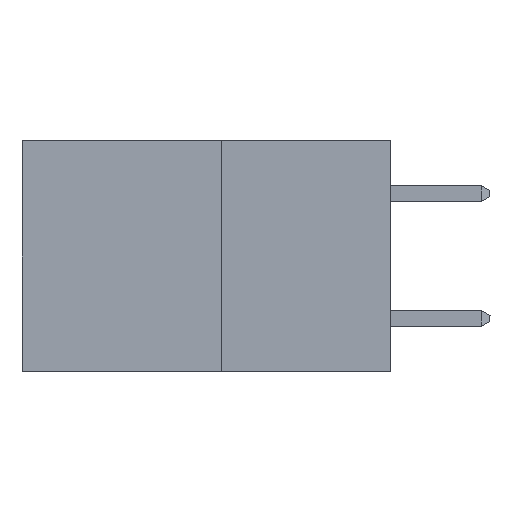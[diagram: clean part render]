
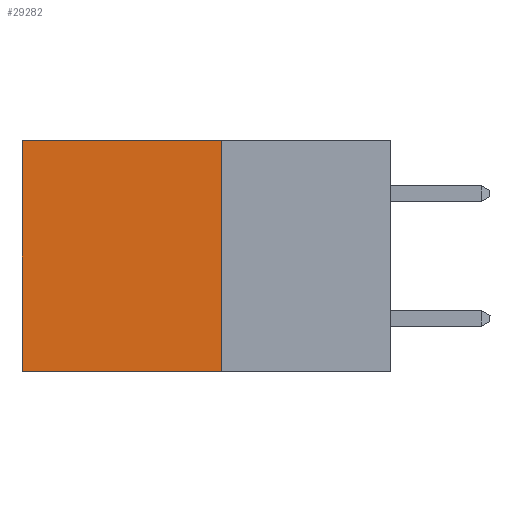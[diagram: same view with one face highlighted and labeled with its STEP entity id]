
A CAD part, left-side view. The second image highlights one B-rep face of the part: STEP entity #29282.
In plain terms, the highlighted planar face has unit normal (-1, 0, 0).
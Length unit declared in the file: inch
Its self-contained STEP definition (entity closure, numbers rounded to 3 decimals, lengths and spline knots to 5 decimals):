
#642 = CARTESIAN_POINT ( 'NONE',  ( 0.277, 0.59, -0.37 ) ) ;
#885 = CARTESIAN_POINT ( 'NONE',  ( 0.277, 0.27, -0.37 ) ) ;
#2436 = VERTEX_POINT ( 'NONE', #17858 ) ;
#3381 = DIRECTION ( 'NONE',  ( 0., 0., -1. ) ) ;
#3770 = AXIS2_PLACEMENT_3D ( 'NONE', #885, #18578, #3381 ) ;
#4627 = CARTESIAN_POINT ( 'NONE',  ( 0.277, 0.27, -0.37 ) ) ;
#4753 = CARTESIAN_POINT ( 'NONE',  ( 0.277, 0.27, 0. ) ) ;
#5964 = DIRECTION ( 'NONE',  ( 0., 0., -1. ) ) ;
#6075 = CARTESIAN_POINT ( 'NONE',  ( 0.277, 0.59, -0.37 ) ) ;
#6175 = VERTEX_POINT ( 'NONE', #27553 ) ;
#6670 = CARTESIAN_POINT ( 'NONE',  ( 0.277, 0.27, -0.37 ) ) ;
#7048 = LINE ( 'NONE', #6075, #19754 ) ;
#7184 = DIRECTION ( 'NONE',  ( 0., 0., -1. ) ) ;
#7358 = ORIENTED_EDGE ( 'NONE', *, *, #10114, .T. ) ;
#10114 = EDGE_CURVE ( 'NONE', #6175, #30348, #7048, .T. ) ;
#13541 = ORIENTED_EDGE ( 'NONE', *, *, #15179, .T. ) ;
#14337 = DIRECTION ( 'NONE',  ( 0., 1., 0. ) ) ;
#15179 = EDGE_CURVE ( 'NONE', #30487, #6175, #24378, .T. ) ;
#16260 = VECTOR ( 'NONE', #7184, 39.37008 ) ;
#17014 = ORIENTED_EDGE ( 'NONE', *, *, #24397, .F. ) ;
#17640 = VECTOR ( 'NONE', #27584, 39.37008 ) ;
#17770 = VECTOR ( 'NONE', #14337, 39.37008 ) ;
#17858 = CARTESIAN_POINT ( 'NONE',  ( 0.277, 0.27, -0.37 ) ) ;
#18578 = DIRECTION ( 'NONE',  ( 1., 0., 0. ) ) ;
#19754 = VECTOR ( 'NONE', #5964, 39.37008 ) ;
#20997 = PLANE ( 'NONE',  #3770 ) ;
#21864 = FACE_OUTER_BOUND ( 'NONE', #25273, .T. ) ;
#24378 = LINE ( 'NONE', #4753, #17640 ) ;
#24397 = EDGE_CURVE ( 'NONE', #30487, #2436, #29751, .T. ) ;
#25273 = EDGE_LOOP ( 'NONE', ( #7358, #27005, #17014, #13541 ) ) ;
#25714 = EDGE_CURVE ( 'NONE', #2436, #30348, #30437, .T. ) ;
#26389 = CARTESIAN_POINT ( 'NONE',  ( 0.277, 0.27, 0. ) ) ;
#27005 = ORIENTED_EDGE ( 'NONE', *, *, #25714, .F. ) ;
#27553 = CARTESIAN_POINT ( 'NONE',  ( 0.277, 0.59, 0. ) ) ;
#27584 = DIRECTION ( 'NONE',  ( 0., 1., 0. ) ) ;
#29282 = ADVANCED_FACE ( 'NONE', ( #21864 ), #20997, .F. ) ;
#29751 = LINE ( 'NONE', #4627, #16260 ) ;
#30348 = VERTEX_POINT ( 'NONE', #642 ) ;
#30437 = LINE ( 'NONE', #6670, #17770 ) ;
#30487 = VERTEX_POINT ( 'NONE', #26389 ) ;
